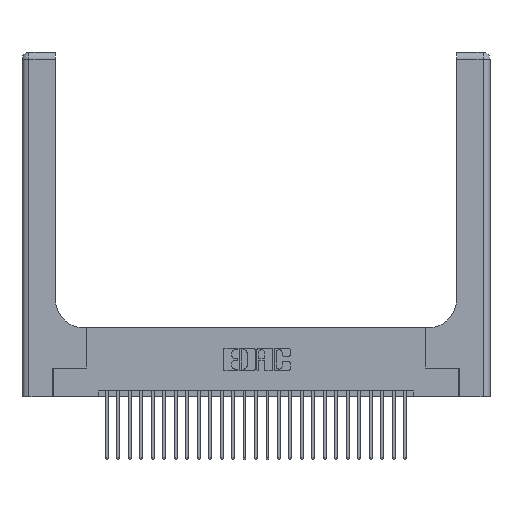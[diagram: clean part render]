
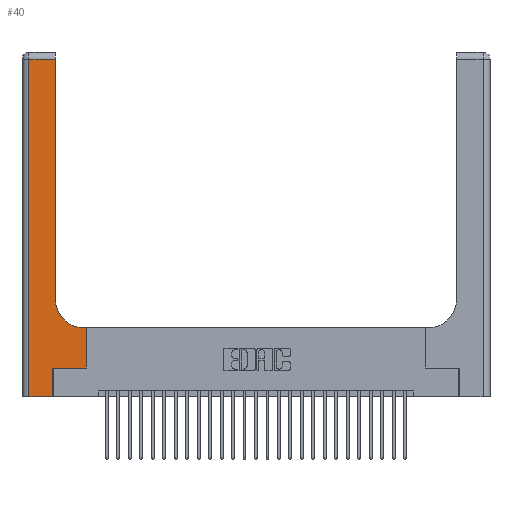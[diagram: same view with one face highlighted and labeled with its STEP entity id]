
A CAD part, top view. The second image highlights one B-rep face of the part: STEP entity #40.
In plain terms, the highlighted planar face has unit normal (0, 0, 1).
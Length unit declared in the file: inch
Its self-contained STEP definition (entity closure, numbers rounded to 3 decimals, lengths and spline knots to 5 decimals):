
#40 = ADVANCED_FACE ( 'NONE', ( #17053 ), #9841, .F. ) ;
#73 = CARTESIAN_POINT ( 'NONE',  ( 0.5415, 0.85, 0.37 ) ) ;
#96 = ORIENTED_EDGE ( 'NONE', *, *, #3031, .T. ) ;
#1741 = CARTESIAN_POINT ( 'NONE',  ( 0.5585, 0.25, 0.37 ) ) ;
#2360 = EDGE_CURVE ( 'NONE', #3693, #17016, #2839, .T. ) ;
#2782 = CARTESIAN_POINT ( 'NONE',  ( 0.2915, 0.85, 0.37 ) ) ;
#2796 = CARTESIAN_POINT ( 'NONE',  ( 0.5585, 0.6, 0.37 ) ) ;
#2839 = LINE ( 'NONE', #13502, #3165 ) ;
#3031 = EDGE_CURVE ( 'NONE', #14493, #3693, #8337, .T. ) ;
#3073 = EDGE_CURVE ( 'NONE', #17016, #14030, #23765, .T. ) ;
#3165 = VECTOR ( 'NONE', #15874, 39.37008 ) ;
#3264 = EDGE_CURVE ( 'NONE', #6550, #10922, #9035, .T. ) ;
#3693 = VERTEX_POINT ( 'NONE', #4329 ) ;
#3748 = LINE ( 'NONE', #24261, #6468 ) ;
#3878 = AXIS2_PLACEMENT_3D ( 'NONE', #6013, #14706, #15099 ) ;
#4329 = CARTESIAN_POINT ( 'NONE',  ( 0.06, 0., 0.37 ) ) ;
#5000 = EDGE_CURVE ( 'NONE', #17748, #10065, #3748, .T. ) ;
#5058 = ORIENTED_EDGE ( 'NONE', *, *, #3073, .T. ) ;
#6013 = CARTESIAN_POINT ( 'NONE',  ( 0., 3., 0.37 ) ) ;
#6458 = CARTESIAN_POINT ( 'NONE',  ( 0.2915, 2.94, 0.37 ) ) ;
#6468 = VECTOR ( 'NONE', #14471, 39.37008 ) ;
#6550 = VERTEX_POINT ( 'NONE', #1741 ) ;
#6916 = VECTOR ( 'NONE', #9743, 39.37008 ) ;
#7727 = LINE ( 'NONE', #16587, #19393 ) ;
#8337 = LINE ( 'NONE', #27513, #17916 ) ;
#9019 = VECTOR ( 'NONE', #11137, 39.37008 ) ;
#9035 = LINE ( 'NONE', #21858, #15856 ) ;
#9544 = DIRECTION ( 'NONE',  ( 1., 0., 0. ) ) ;
#9743 = DIRECTION ( 'NONE',  ( 0., 1., 0. ) ) ;
#9841 = PLANE ( 'NONE',  #3878 ) ;
#10065 = VERTEX_POINT ( 'NONE', #6458 ) ;
#10116 = VECTOR ( 'NONE', #9544, 39.37008 ) ;
#10841 = CARTESIAN_POINT ( 'NONE',  ( 0.269, 0.25, 0.37 ) ) ;
#10922 = VERTEX_POINT ( 'NONE', #2796 ) ;
#11137 = DIRECTION ( 'NONE',  ( -1., 0., 0. ) ) ;
#11523 = ORIENTED_EDGE ( 'NONE', *, *, #2360, .T. ) ;
#12332 = CARTESIAN_POINT ( 'NONE',  ( 0.269, 0., 0.37 ) ) ;
#13502 = CARTESIAN_POINT ( 'NONE',  ( 0., 0., 0.37 ) ) ;
#13666 = CARTESIAN_POINT ( 'NONE',  ( 0.269, 0.25, 0.37 ) ) ;
#13673 = EDGE_CURVE ( 'NONE', #20738, #17748, #16092, .T. ) ;
#14030 = VERTEX_POINT ( 'NONE', #10841 ) ;
#14230 = ORIENTED_EDGE ( 'NONE', *, *, #16510, .T. ) ;
#14234 = ORIENTED_EDGE ( 'NONE', *, *, #15771, .T. ) ;
#14471 = DIRECTION ( 'NONE',  ( 0., 1., 0. ) ) ;
#14493 = VERTEX_POINT ( 'NONE', #18198 ) ;
#14706 = DIRECTION ( 'NONE',  ( 0., 0., -1. ) ) ;
#15090 = DIRECTION ( 'NONE',  ( 0., 0., -1. ) ) ;
#15099 = DIRECTION ( 'NONE',  ( -1., 0., 0. ) ) ;
#15462 = DIRECTION ( 'NONE',  ( 1., 0., 0. ) ) ;
#15771 = EDGE_CURVE ( 'NONE', #10065, #14493, #7727, .T. ) ;
#15856 = VECTOR ( 'NONE', #23896, 39.37008 ) ;
#15872 = LINE ( 'NONE', #21737, #9019 ) ;
#15874 = DIRECTION ( 'NONE',  ( 1., 0., 0. ) ) ;
#16092 = CIRCLE ( 'NONE', #23625, 0.25 ) ;
#16510 = EDGE_CURVE ( 'NONE', #14030, #6550, #22450, .T. ) ;
#16587 = CARTESIAN_POINT ( 'NONE',  ( 0., 2.94, 0.37 ) ) ;
#16613 = ORIENTED_EDGE ( 'NONE', *, *, #3264, .T. ) ;
#17016 = VERTEX_POINT ( 'NONE', #17248 ) ;
#17053 = FACE_OUTER_BOUND ( 'NONE', #27311, .T. ) ;
#17248 = CARTESIAN_POINT ( 'NONE',  ( 0.269, 0., 0.37 ) ) ;
#17299 = EDGE_CURVE ( 'NONE', #10922, #20738, #15872, .T. ) ;
#17748 = VERTEX_POINT ( 'NONE', #2782 ) ;
#17916 = VECTOR ( 'NONE', #18523, 39.37008 ) ;
#18198 = CARTESIAN_POINT ( 'NONE',  ( 0.06, 2.94, 0.37 ) ) ;
#18417 = ORIENTED_EDGE ( 'NONE', *, *, #5000, .T. ) ;
#18516 = ORIENTED_EDGE ( 'NONE', *, *, #17299, .T. ) ;
#18523 = DIRECTION ( 'NONE',  ( 0., -1., 0. ) ) ;
#19393 = VECTOR ( 'NONE', #23205, 39.37008 ) ;
#20738 = VERTEX_POINT ( 'NONE', #26023 ) ;
#21737 = CARTESIAN_POINT ( 'NONE',  ( 0.2915, 0.6, 0.37 ) ) ;
#21858 = CARTESIAN_POINT ( 'NONE',  ( 0.5585, 0.25, 0.37 ) ) ;
#22450 = LINE ( 'NONE', #13666, #10116 ) ;
#23205 = DIRECTION ( 'NONE',  ( -1., 0., 0. ) ) ;
#23625 = AXIS2_PLACEMENT_3D ( 'NONE', #73, #15090, #15462 ) ;
#23765 = LINE ( 'NONE', #12332, #6916 ) ;
#23842 = ORIENTED_EDGE ( 'NONE', *, *, #13673, .T. ) ;
#23896 = DIRECTION ( 'NONE',  ( 0., 1., 0. ) ) ;
#24261 = CARTESIAN_POINT ( 'NONE',  ( 0.2915, 3., 0.37 ) ) ;
#26023 = CARTESIAN_POINT ( 'NONE',  ( 0.5415, 0.6, 0.37 ) ) ;
#27311 = EDGE_LOOP ( 'NONE', ( #18417, #14234, #96, #11523, #5058, #14230, #16613, #18516, #23842 ) ) ;
#27513 = CARTESIAN_POINT ( 'NONE',  ( 0.06, 3., 0.37 ) ) ;
